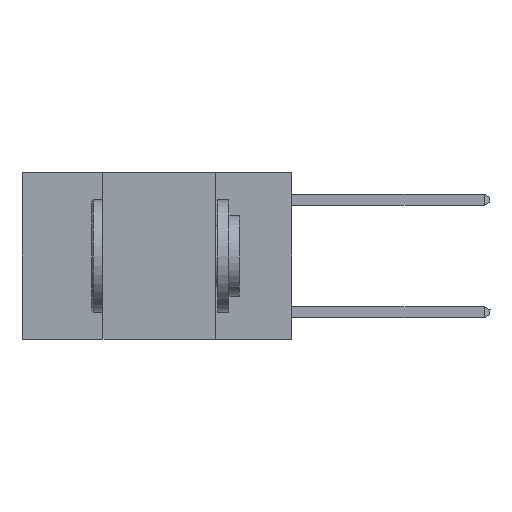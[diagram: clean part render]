
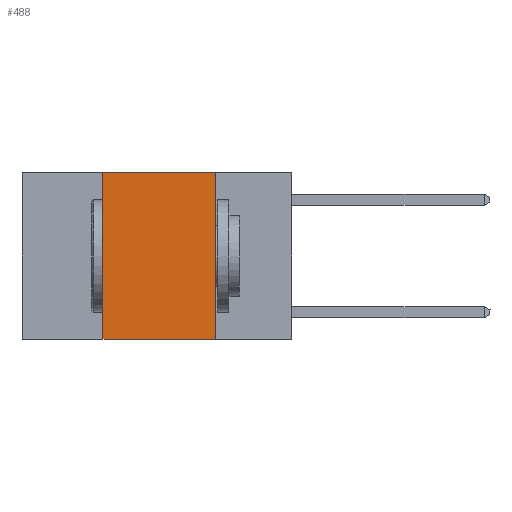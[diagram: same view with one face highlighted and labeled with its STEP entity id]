
A CAD part, left-side view. The second image highlights one B-rep face of the part: STEP entity #488.
In plain terms, the highlighted planar face has unit normal (-1, 0, 0).
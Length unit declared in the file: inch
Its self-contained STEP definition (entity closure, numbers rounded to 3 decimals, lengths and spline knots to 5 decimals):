
#268 = VECTOR ( 'NONE', #16833, 39.37008 ) ;
#488 = ADVANCED_FACE ( 'NONE', ( #3112 ), #21776, .F. ) ;
#1260 = LINE ( 'NONE', #11925, #23197 ) ;
#1951 = EDGE_LOOP ( 'NONE', ( #16275, #17002, #17674, #17828 ) ) ;
#3112 = FACE_OUTER_BOUND ( 'NONE', #1951, .T. ) ;
#3115 = LINE ( 'NONE', #5447, #19517 ) ;
#3399 = CARTESIAN_POINT ( 'NONE',  ( 0., 0.42, -0.37 ) ) ;
#3840 = LINE ( 'NONE', #12820, #10304 ) ;
#4463 = VERTEX_POINT ( 'NONE', #15335 ) ;
#5447 = CARTESIAN_POINT ( 'NONE',  ( 0., 0.6, 0. ) ) ;
#6313 = DIRECTION ( 'NONE',  ( 0., 0., -1. ) ) ;
#6320 = LINE ( 'NONE', #24755, #268 ) ;
#6420 = EDGE_CURVE ( 'NONE', #9227, #14861, #6320, .T. ) ;
#9090 = AXIS2_PLACEMENT_3D ( 'NONE', #17773, #23758, #11449 ) ;
#9227 = VERTEX_POINT ( 'NONE', #3399 ) ;
#10304 = VECTOR ( 'NONE', #6313, 39.37008 ) ;
#11449 = DIRECTION ( 'NONE',  ( 0., 0., -1. ) ) ;
#11547 = CARTESIAN_POINT ( 'NONE',  ( 0., 0.17, -0.37 ) ) ;
#11925 = CARTESIAN_POINT ( 'NONE',  ( 0., 0.42, 0. ) ) ;
#12820 = CARTESIAN_POINT ( 'NONE',  ( 0., 0.17, 0. ) ) ;
#14861 = VERTEX_POINT ( 'NONE', #11547 ) ;
#15335 = CARTESIAN_POINT ( 'NONE',  ( 0., 0.42, 0. ) ) ;
#16275 = ORIENTED_EDGE ( 'NONE', *, *, #19191, .F. ) ;
#16833 = DIRECTION ( 'NONE',  ( 0., -1., 0. ) ) ;
#17002 = ORIENTED_EDGE ( 'NONE', *, *, #25184, .F. ) ;
#17674 = ORIENTED_EDGE ( 'NONE', *, *, #20526, .F. ) ;
#17773 = CARTESIAN_POINT ( 'NONE',  ( 0., 0.6, 0. ) ) ;
#17828 = ORIENTED_EDGE ( 'NONE', *, *, #6420, .T. ) ;
#18254 = DIRECTION ( 'NONE',  ( 0., -1., 0. ) ) ;
#19191 = EDGE_CURVE ( 'NONE', #26348, #14861, #3840, .T. ) ;
#19517 = VECTOR ( 'NONE', #18254, 39.37008 ) ;
#20526 = EDGE_CURVE ( 'NONE', #9227, #4463, #1260, .T. ) ;
#21776 = PLANE ( 'NONE',  #9090 ) ;
#23197 = VECTOR ( 'NONE', #24170, 39.37008 ) ;
#23758 = DIRECTION ( 'NONE',  ( 1., 0., 0. ) ) ;
#24170 = DIRECTION ( 'NONE',  ( 0., 0., 1. ) ) ;
#24755 = CARTESIAN_POINT ( 'NONE',  ( 0., 0.6, -0.37 ) ) ;
#24869 = CARTESIAN_POINT ( 'NONE',  ( 0., 0.17, 0. ) ) ;
#25184 = EDGE_CURVE ( 'NONE', #4463, #26348, #3115, .T. ) ;
#26348 = VERTEX_POINT ( 'NONE', #24869 ) ;
